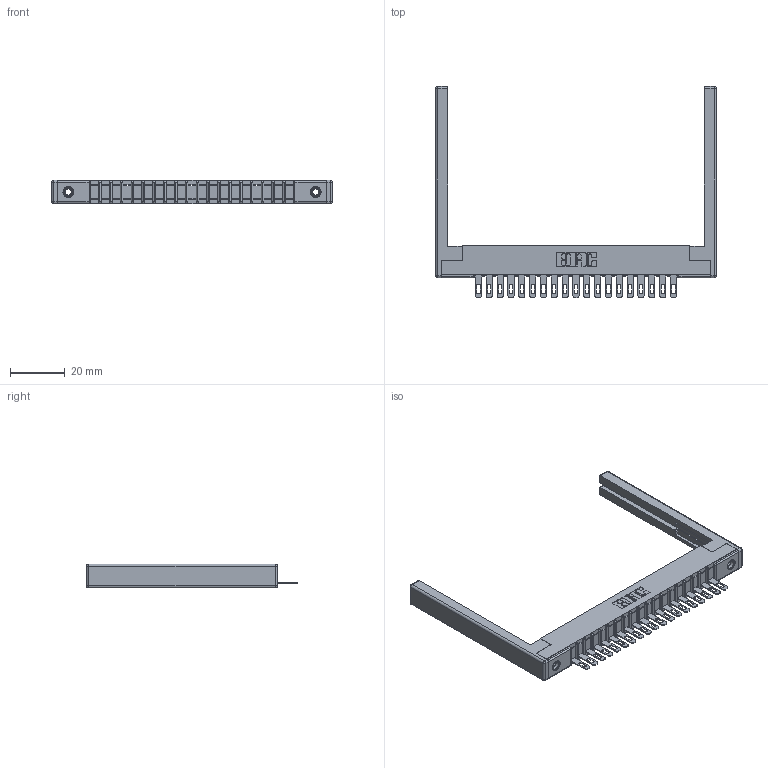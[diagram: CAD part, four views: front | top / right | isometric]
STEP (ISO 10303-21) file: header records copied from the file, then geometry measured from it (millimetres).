
FILE_DESCRIPTION (( 'STEP AP203' ), '1' );
FILE_NAME ('357-019-505-168.STEP', '2019-09-13T22:30:03', ( '' ), ( '' ), 'SwSTEP 2.0', 'SolidWorks 2016', '' );
FILE_SCHEMA (( 'CONFIG_CONTROL_DESIGN' ));
Length unit declared in the file: inch
Products named in the file (5): 307-290-001_505; 345-250-001_345-250-001-102; 307 Part_.156 Dia Mounting Holes; 307-220-068; 357-019-505-168
Assembly tree (24 placements, depth 2):
  357-019-505-168
    307 Part_.156 Dia Mounting Holes
    307-290-001_505  x19
    307-220-068  x2
    345-250-001_345-250-001-102  x2
Bounding box: 102.72 x 77.14 x 8.71 mm (x, y, z)
Volume: 11089.9 mm3; surface area: 14273.3 mm2
Topology: 24 solids, 24 shells, 1356 faces, 3791 edges, 2426 vertices
Faces by surface type: plane 842, cylinder 450, sphere 48, cone 12, torus 4
Entity records: 21857 total; most frequent: CARTESIAN_POINT 3637, ORIENTED_EDGE 3612, DIRECTION 3570, EDGE_CURVE 1806, LINE 1372, VECTOR 1372, VERTEX_POINT 1166, AXIS2_PLACEMENT_3D 1099
